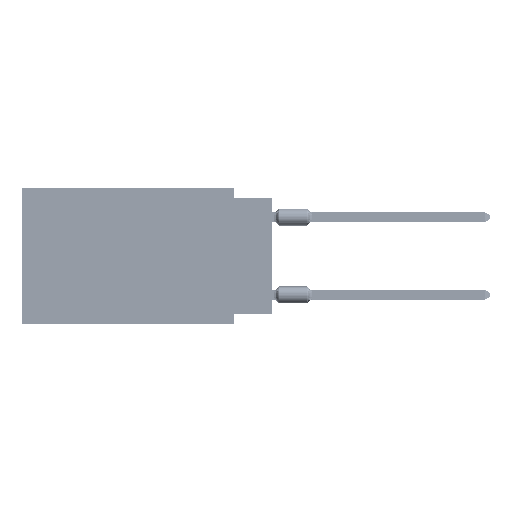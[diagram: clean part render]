
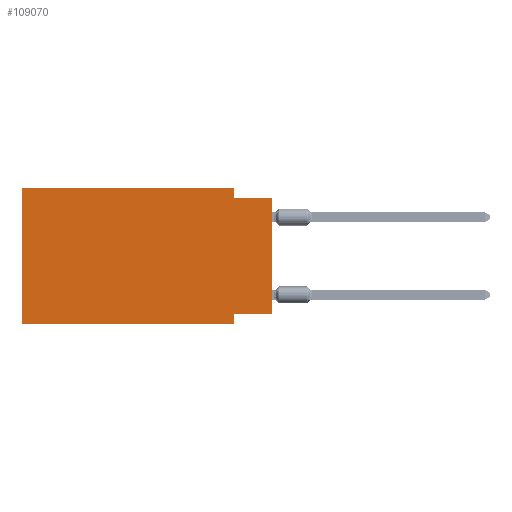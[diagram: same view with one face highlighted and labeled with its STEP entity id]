
A CAD part, left-side view. The second image highlights one B-rep face of the part: STEP entity #109070.
In plain terms, the highlighted planar face has unit normal (-1, 0, 0).
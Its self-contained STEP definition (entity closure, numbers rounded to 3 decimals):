
#2283 = CARTESIAN_POINT ( 'NONE',  ( 0., 16.383, 0. ) ) ;
#3837 = CARTESIAN_POINT ( 'NONE',  ( 0., 16.383, 0. ) ) ;
#5151 = DIRECTION ( 'NONE',  ( 0., 0., -1. ) ) ;
#6376 = LINE ( 'NONE', #117820, #39718 ) ;
#9881 = EDGE_CURVE ( 'NONE', #103630, #51879, #71048, .T. ) ;
#10474 = EDGE_CURVE ( 'NONE', #73438, #95208, #109686, .T. ) ;
#11527 = FACE_OUTER_BOUND ( 'NONE', #14319, .T. ) ;
#11875 = LINE ( 'NONE', #3837, #77499 ) ;
#12130 = VERTEX_POINT ( 'NONE', #100308 ) ;
#14319 = EDGE_LOOP ( 'NONE', ( #83438, #32524, #50446, #117935, #96887, #14743, #106586, #106856 ) ) ;
#14743 = ORIENTED_EDGE ( 'NONE', *, *, #76153, .T. ) ;
#14836 = DIRECTION ( 'NONE',  ( 0., 1., 0. ) ) ;
#18453 = CARTESIAN_POINT ( 'NONE',  ( 0., 16.383, -8.89 ) ) ;
#25148 = EDGE_CURVE ( 'NONE', #95208, #81422, #6376, .T. ) ;
#32524 = ORIENTED_EDGE ( 'NONE', *, *, #9881, .F. ) ;
#33285 = EDGE_CURVE ( 'NONE', #100406, #12130, #11875, .T. ) ;
#34150 = CARTESIAN_POINT ( 'NONE',  ( 0., 2.54, 0. ) ) ;
#35731 = DIRECTION ( 'NONE',  ( 0., 0., 1. ) ) ;
#36343 = LINE ( 'NONE', #103469, #86398 ) ;
#36673 = CARTESIAN_POINT ( 'NONE',  ( 0., 2.54, -8.255 ) ) ;
#39718 = VECTOR ( 'NONE', #5151, 1000. ) ;
#39868 = DIRECTION ( 'NONE',  ( 0., 0., -1. ) ) ;
#40907 = CARTESIAN_POINT ( 'NONE',  ( 0., 0., -0.635 ) ) ;
#41999 = DIRECTION ( 'NONE',  ( 0., 0., 1. ) ) ;
#44867 = EDGE_CURVE ( 'NONE', #12130, #103630, #107457, .T. ) ;
#44956 = CARTESIAN_POINT ( 'NONE',  ( 0., 2.54, -0.635 ) ) ;
#47158 = VECTOR ( 'NONE', #14836, 1000. ) ;
#50446 = ORIENTED_EDGE ( 'NONE', *, *, #44867, .F. ) ;
#51879 = VERTEX_POINT ( 'NONE', #53760 ) ;
#53760 = CARTESIAN_POINT ( 'NONE',  ( 0., 0., -0.635 ) ) ;
#54228 = VECTOR ( 'NONE', #90804, 1000. ) ;
#55176 = DIRECTION ( 'NONE',  ( 0., -1., 0. ) ) ;
#58210 = VECTOR ( 'NONE', #41999, 1000. ) ;
#62306 = VERTEX_POINT ( 'NONE', #18453 ) ;
#62335 = CARTESIAN_POINT ( 'NONE',  ( 0., 16.383, 0. ) ) ;
#71048 = LINE ( 'NONE', #40907, #111977 ) ;
#73438 = VERTEX_POINT ( 'NONE', #117727 ) ;
#76153 = EDGE_CURVE ( 'NONE', #62306, #81422, #109422, .T. ) ;
#77499 = VECTOR ( 'NONE', #78971, 1000. ) ;
#78034 = DIRECTION ( 'NONE',  ( 1., 0., 0. ) ) ;
#78971 = DIRECTION ( 'NONE',  ( 0., -1., 0. ) ) ;
#80180 = LINE ( 'NONE', #115921, #58210 ) ;
#81422 = VERTEX_POINT ( 'NONE', #100892 ) ;
#83438 = ORIENTED_EDGE ( 'NONE', *, *, #85622, .T. ) ;
#85622 = EDGE_CURVE ( 'NONE', #73438, #51879, #80180, .T. ) ;
#86398 = VECTOR ( 'NONE', #35731, 1000. ) ;
#90804 = DIRECTION ( 'NONE',  ( 0., 0., -1. ) ) ;
#93080 = EDGE_CURVE ( 'NONE', #62306, #100406, #36343, .T. ) ;
#95208 = VERTEX_POINT ( 'NONE', #36673 ) ;
#96887 = ORIENTED_EDGE ( 'NONE', *, *, #93080, .F. ) ;
#97187 = VECTOR ( 'NONE', #55176, 1000. ) ;
#98380 = AXIS2_PLACEMENT_3D ( 'NONE', #2283, #78034, #39868 ) ;
#100308 = CARTESIAN_POINT ( 'NONE',  ( 0., 2.54, 0. ) ) ;
#100406 = VERTEX_POINT ( 'NONE', #62335 ) ;
#100892 = CARTESIAN_POINT ( 'NONE',  ( 0., 2.54, -8.89 ) ) ;
#103469 = CARTESIAN_POINT ( 'NONE',  ( 0., 16.383, 0. ) ) ;
#103630 = VERTEX_POINT ( 'NONE', #44956 ) ;
#106586 = ORIENTED_EDGE ( 'NONE', *, *, #25148, .F. ) ;
#106802 = DIRECTION ( 'NONE',  ( 0., -1., 0. ) ) ;
#106856 = ORIENTED_EDGE ( 'NONE', *, *, #10474, .F. ) ;
#107457 = LINE ( 'NONE', #34150, #54228 ) ;
#109070 = ADVANCED_FACE ( 'NONE', ( #11527 ), #117389, .F. ) ;
#109422 = LINE ( 'NONE', #111241, #97187 ) ;
#109686 = LINE ( 'NONE', #120752, #47158 ) ;
#111241 = CARTESIAN_POINT ( 'NONE',  ( 0., 16.383, -8.89 ) ) ;
#111977 = VECTOR ( 'NONE', #106802, 1000. ) ;
#115921 = CARTESIAN_POINT ( 'NONE',  ( 0., 0., 0. ) ) ;
#117389 = PLANE ( 'NONE',  #98380 ) ;
#117727 = CARTESIAN_POINT ( 'NONE',  ( 0., 0., -8.255 ) ) ;
#117820 = CARTESIAN_POINT ( 'NONE',  ( 0., 2.54, -8.89 ) ) ;
#117935 = ORIENTED_EDGE ( 'NONE', *, *, #33285, .F. ) ;
#120752 = CARTESIAN_POINT ( 'NONE',  ( 0., 0., -8.255 ) ) ;
